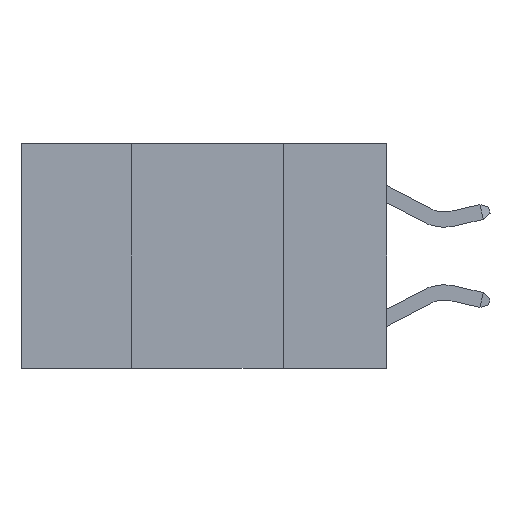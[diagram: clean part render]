
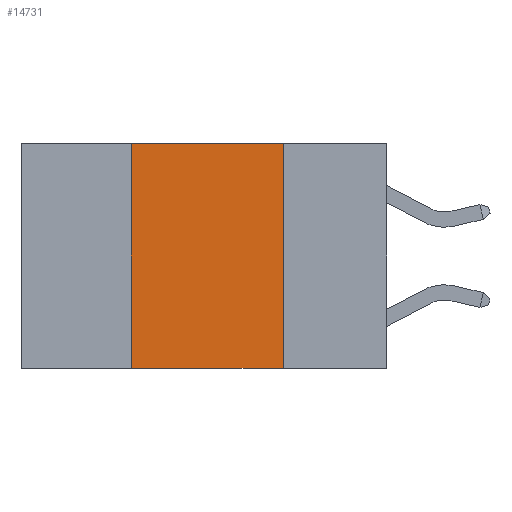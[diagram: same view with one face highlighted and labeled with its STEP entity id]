
A CAD part, left-side view. The second image highlights one B-rep face of the part: STEP entity #14731.
In plain terms, the highlighted planar face has unit normal (-1, 0, 0).
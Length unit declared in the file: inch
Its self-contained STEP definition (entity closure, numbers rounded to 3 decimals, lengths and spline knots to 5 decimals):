
#122 = VECTOR ( 'NONE', #9940, 39.37008 ) ;
#695 = CARTESIAN_POINT ( 'NONE',  ( 0., 0.6, 0. ) ) ;
#1067 = LINE ( 'NONE', #695, #12007 ) ;
#2278 = VERTEX_POINT ( 'NONE', #16664 ) ;
#2533 = EDGE_CURVE ( 'NONE', #9815, #13361, #12020, .T. ) ;
#2611 = DIRECTION ( 'NONE',  ( 0., 0., 1. ) ) ;
#2878 = VECTOR ( 'NONE', #8265, 39.37008 ) ;
#3085 = DIRECTION ( 'NONE',  ( 0., 0., -1. ) ) ;
#3724 = EDGE_CURVE ( 'NONE', #9570, #9815, #1067, .T. ) ;
#4135 = CARTESIAN_POINT ( 'NONE',  ( 0., 0.42, 0. ) ) ;
#4649 = LINE ( 'NONE', #4135, #15931 ) ;
#4692 = ORIENTED_EDGE ( 'NONE', *, *, #2533, .F. ) ;
#5569 = CARTESIAN_POINT ( 'NONE',  ( 0., 0.17, 0. ) ) ;
#5646 = ORIENTED_EDGE ( 'NONE', *, *, #7927, .F. ) ;
#6040 = CARTESIAN_POINT ( 'NONE',  ( 0., 0.6, 0. ) ) ;
#6790 = CARTESIAN_POINT ( 'NONE',  ( 0., 0.6, -0.37 ) ) ;
#7280 = CARTESIAN_POINT ( 'NONE',  ( 0., 0.17, 0. ) ) ;
#7927 = EDGE_CURVE ( 'NONE', #2278, #9570, #4649, .T. ) ;
#8265 = DIRECTION ( 'NONE',  ( 0., -1., 0. ) ) ;
#8994 = PLANE ( 'NONE',  #14266 ) ;
#9094 = ORIENTED_EDGE ( 'NONE', *, *, #3724, .F. ) ;
#9570 = VERTEX_POINT ( 'NONE', #16731 ) ;
#9637 = DIRECTION ( 'NONE',  ( 0., -1., 0. ) ) ;
#9815 = VERTEX_POINT ( 'NONE', #7280 ) ;
#9940 = DIRECTION ( 'NONE',  ( 0., 0., -1. ) ) ;
#10982 = EDGE_CURVE ( 'NONE', #2278, #13361, #14689, .T. ) ;
#11940 = CARTESIAN_POINT ( 'NONE',  ( 0., 0.17, -0.37 ) ) ;
#11957 = DIRECTION ( 'NONE',  ( 1., 0., 0. ) ) ;
#12007 = VECTOR ( 'NONE', #9637, 39.37008 ) ;
#12020 = LINE ( 'NONE', #5569, #122 ) ;
#12399 = EDGE_LOOP ( 'NONE', ( #4692, #9094, #5646, #13486 ) ) ;
#13361 = VERTEX_POINT ( 'NONE', #11940 ) ;
#13486 = ORIENTED_EDGE ( 'NONE', *, *, #10982, .T. ) ;
#14266 = AXIS2_PLACEMENT_3D ( 'NONE', #6040, #11957, #3085 ) ;
#14689 = LINE ( 'NONE', #6790, #2878 ) ;
#14731 = ADVANCED_FACE ( 'NONE', ( #19113 ), #8994, .F. ) ;
#15931 = VECTOR ( 'NONE', #2611, 39.37008 ) ;
#16664 = CARTESIAN_POINT ( 'NONE',  ( 0., 0.42, -0.37 ) ) ;
#16731 = CARTESIAN_POINT ( 'NONE',  ( 0., 0.42, 0. ) ) ;
#19113 = FACE_OUTER_BOUND ( 'NONE', #12399, .T. ) ;
